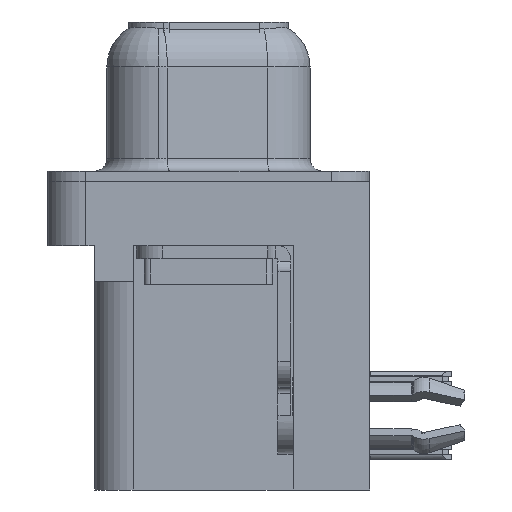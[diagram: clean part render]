
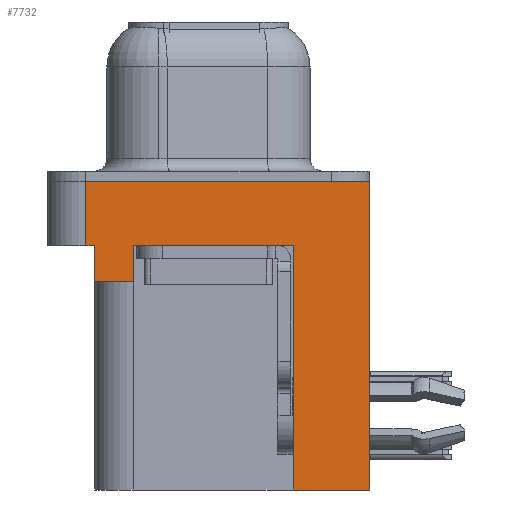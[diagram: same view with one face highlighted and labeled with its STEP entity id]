
A CAD part, left-side view. The second image highlights one B-rep face of the part: STEP entity #7732.
In plain terms, the highlighted planar face has unit normal (-1, 0, 0).
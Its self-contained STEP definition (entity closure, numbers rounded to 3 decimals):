
#54 = LINE ( 'NONE', #29560, #6365 ) ;
#287 = EDGE_CURVE ( 'NONE', #5359, #32640, #13022, .T. ) ;
#567 = VERTEX_POINT ( 'NONE', #11729 ) ;
#658 = EDGE_CURVE ( 'NONE', #20493, #567, #6284, .T. ) ;
#902 = VECTOR ( 'NONE', #21114, 1000. ) ;
#1411 = LINE ( 'NONE', #6527, #5326 ) ;
#1761 = DIRECTION ( 'NONE',  ( 0., -1., 0. ) ) ;
#2017 = DIRECTION ( 'NONE',  ( 0., -1., 0. ) ) ;
#2400 = VECTOR ( 'NONE', #2017, 1000. ) ;
#3615 = DIRECTION ( 'NONE',  ( -1., 0., 0. ) ) ;
#3910 = VECTOR ( 'NONE', #32157, 1000. ) ;
#5326 = VECTOR ( 'NONE', #6859, 1000. ) ;
#5359 = VERTEX_POINT ( 'NONE', #23493 ) ;
#5835 = VERTEX_POINT ( 'NONE', #16546 ) ;
#6004 = PLANE ( 'NONE',  #11609 ) ;
#6284 = LINE ( 'NONE', #27597, #3910 ) ;
#6365 = VECTOR ( 'NONE', #1761, 1000. ) ;
#6527 = CARTESIAN_POINT ( 'NONE',  ( -3., -6.275, 0. ) ) ;
#6859 = DIRECTION ( 'NONE',  ( 0., -1., 0. ) ) ;
#7674 = EDGE_CURVE ( 'NONE', #12131, #17310, #12423, .T. ) ;
#7732 = ADVANCED_FACE ( 'NONE', ( #26712 ), #6004, .T. ) ;
#7764 = DIRECTION ( 'NONE',  ( 0., 1., 0. ) ) ;
#8781 = CARTESIAN_POINT ( 'NONE',  ( -3., -6.275, -2.5 ) ) ;
#9630 = VECTOR ( 'NONE', #13541, 1000. ) ;
#9856 = EDGE_CURVE ( 'NONE', #32640, #5835, #23436, .T. ) ;
#9916 = EDGE_CURVE ( 'NONE', #16318, #26487, #54, .T. ) ;
#10543 = CARTESIAN_POINT ( 'NONE',  ( -3., -3.295, -12. ) ) ;
#11192 = EDGE_LOOP ( 'NONE', ( #30728, #27462, #28531, #20226, #27590, #26958, #14248, #20219, #21964, #27935 ) ) ;
#11609 = AXIS2_PLACEMENT_3D ( 'NONE', #8781, #3615, #24140 ) ;
#11622 = DIRECTION ( 'NONE',  ( 0., 0., 1. ) ) ;
#11729 = CARTESIAN_POINT ( 'NONE',  ( -3., 4.775, 0. ) ) ;
#11993 = VECTOR ( 'NONE', #27593, 1000. ) ;
#12131 = VERTEX_POINT ( 'NONE', #18298 ) ;
#12423 = LINE ( 'NONE', #10543, #9630 ) ;
#12508 = CARTESIAN_POINT ( 'NONE',  ( -3., -6.275, 0. ) ) ;
#13022 = LINE ( 'NONE', #25318, #32391 ) ;
#13426 = LINE ( 'NONE', #14468, #2400 ) ;
#13506 = CARTESIAN_POINT ( 'NONE',  ( -3., 2.895, -3.9 ) ) ;
#13541 = DIRECTION ( 'NONE',  ( 0., 1., 0. ) ) ;
#14248 = ORIENTED_EDGE ( 'NONE', *, *, #9916, .T. ) ;
#14468 = CARTESIAN_POINT ( 'NONE',  ( -3., -6.275, -2.5 ) ) ;
#14660 = CARTESIAN_POINT ( 'NONE',  ( -3., -3.295, -12. ) ) ;
#15447 = CARTESIAN_POINT ( 'NONE',  ( -3., -3.295, -2.5 ) ) ;
#16318 = VERTEX_POINT ( 'NONE', #23003 ) ;
#16546 = CARTESIAN_POINT ( 'NONE',  ( -3., 4.425, -2.5 ) ) ;
#17310 = VERTEX_POINT ( 'NONE', #18239 ) ;
#18239 = CARTESIAN_POINT ( 'NONE',  ( -3., -3.295, -12. ) ) ;
#18298 = CARTESIAN_POINT ( 'NONE',  ( -3., -6.275, -12. ) ) ;
#20219 = ORIENTED_EDGE ( 'NONE', *, *, #29954, .F. ) ;
#20226 = ORIENTED_EDGE ( 'NONE', *, *, #9856, .F. ) ;
#20299 = CARTESIAN_POINT ( 'NONE',  ( -3., -6.275, -2.5 ) ) ;
#20493 = VERTEX_POINT ( 'NONE', #25505 ) ;
#20855 = EDGE_CURVE ( 'NONE', #567, #24049, #1411, .T. ) ;
#21114 = DIRECTION ( 'NONE',  ( 0., 0., 1. ) ) ;
#21964 = ORIENTED_EDGE ( 'NONE', *, *, #7674, .F. ) ;
#22272 = LINE ( 'NONE', #13506, #902 ) ;
#23003 = CARTESIAN_POINT ( 'NONE',  ( -3., 2.895, -2.5 ) ) ;
#23436 = LINE ( 'NONE', #28101, #24201 ) ;
#23493 = CARTESIAN_POINT ( 'NONE',  ( -3., 2.895, -3.9 ) ) ;
#24049 = VERTEX_POINT ( 'NONE', #12508 ) ;
#24140 = DIRECTION ( 'NONE',  ( 0., 0., 1. ) ) ;
#24201 = VECTOR ( 'NONE', #11622, 1000. ) ;
#25318 = CARTESIAN_POINT ( 'NONE',  ( -3., 4.425, -3.9 ) ) ;
#25505 = CARTESIAN_POINT ( 'NONE',  ( -3., 4.775, -2.5 ) ) ;
#26487 = VERTEX_POINT ( 'NONE', #15447 ) ;
#26565 = LINE ( 'NONE', #20299, #11993 ) ;
#26712 = FACE_OUTER_BOUND ( 'NONE', #11192, .T. ) ;
#26958 = ORIENTED_EDGE ( 'NONE', *, *, #27602, .T. ) ;
#27462 = ORIENTED_EDGE ( 'NONE', *, *, #658, .F. ) ;
#27590 = ORIENTED_EDGE ( 'NONE', *, *, #287, .F. ) ;
#27593 = DIRECTION ( 'NONE',  ( 0., 0., 1. ) ) ;
#27597 = CARTESIAN_POINT ( 'NONE',  ( -3., 4.775, -2.5 ) ) ;
#27602 = EDGE_CURVE ( 'NONE', #5359, #16318, #22272, .T. ) ;
#27778 = EDGE_CURVE ( 'NONE', #12131, #24049, #26565, .T. ) ;
#27935 = ORIENTED_EDGE ( 'NONE', *, *, #27778, .T. ) ;
#28101 = CARTESIAN_POINT ( 'NONE',  ( -3., 4.425, -3.9 ) ) ;
#28531 = ORIENTED_EDGE ( 'NONE', *, *, #30398, .T. ) ;
#29560 = CARTESIAN_POINT ( 'NONE',  ( -3., -6.275, -2.5 ) ) ;
#29779 = CARTESIAN_POINT ( 'NONE',  ( -3., 4.425, -3.9 ) ) ;
#29954 = EDGE_CURVE ( 'NONE', #17310, #26487, #30830, .T. ) ;
#30398 = EDGE_CURVE ( 'NONE', #20493, #5835, #13426, .T. ) ;
#30448 = VECTOR ( 'NONE', #32359, 1000. ) ;
#30728 = ORIENTED_EDGE ( 'NONE', *, *, #20855, .F. ) ;
#30830 = LINE ( 'NONE', #14660, #30448 ) ;
#32157 = DIRECTION ( 'NONE',  ( 0., 0., 1. ) ) ;
#32359 = DIRECTION ( 'NONE',  ( 0., 0., 1. ) ) ;
#32391 = VECTOR ( 'NONE', #7764, 1000. ) ;
#32640 = VERTEX_POINT ( 'NONE', #29779 ) ;
